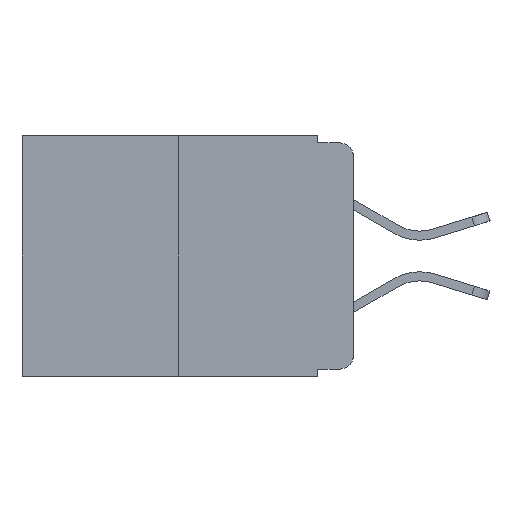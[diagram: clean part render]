
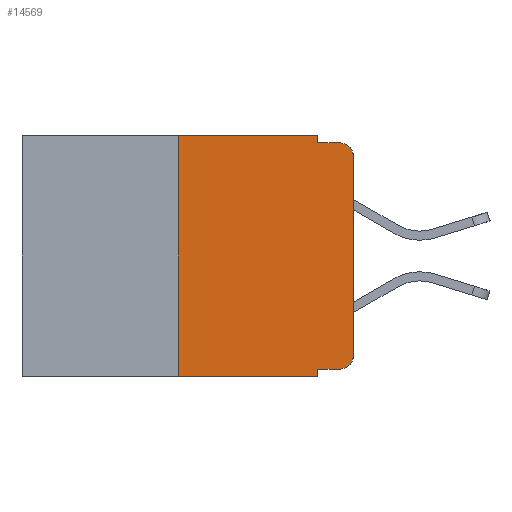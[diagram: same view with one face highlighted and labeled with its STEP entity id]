
A CAD part, left-side view. The second image highlights one B-rep face of the part: STEP entity #14569.
In plain terms, the highlighted planar face has unit normal (-1, 0, 0).
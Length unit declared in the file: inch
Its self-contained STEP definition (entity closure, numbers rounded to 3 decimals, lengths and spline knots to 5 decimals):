
#28 = VECTOR ( 'NONE', #1936, 39.37008 ) ;
#197 = DIRECTION ( 'NONE',  ( 0., 0., -1. ) ) ;
#256 = CARTESIAN_POINT ( 'NONE',  ( 0., 0.02, -0.313 ) ) ;
#475 = VECTOR ( 'NONE', #15218, 39.37008 ) ;
#536 = PLANE ( 'NONE',  #572 ) ;
#572 = AXIS2_PLACEMENT_3D ( 'NONE', #13482, #4297, #12432 ) ;
#718 = EDGE_CURVE ( 'NONE', #2186, #5644, #10550, .T. ) ;
#736 = VERTEX_POINT ( 'NONE', #10210 ) ;
#752 = LINE ( 'NONE', #10221, #3677 ) ;
#781 = LINE ( 'NONE', #7168, #12965 ) ;
#795 = ORIENTED_EDGE ( 'NONE', *, *, #718, .T. ) ;
#831 = ORIENTED_EDGE ( 'NONE', *, *, #15114, .T. ) ;
#867 = ORIENTED_EDGE ( 'NONE', *, *, #14377, .F. ) ;
#888 = ORIENTED_EDGE ( 'NONE', *, *, #13630, .F. ) ;
#1023 = ORIENTED_EDGE ( 'NONE', *, *, #5543, .F. ) ;
#1114 = ORIENTED_EDGE ( 'NONE', *, *, #12880, .F. ) ;
#1164 = ORIENTED_EDGE ( 'NONE', *, *, #5335, .T. ) ;
#1300 = ORIENTED_EDGE ( 'NONE', *, *, #12161, .F. ) ;
#1325 = ORIENTED_EDGE ( 'NONE', *, *, #11409, .T. ) ;
#1339 = ORIENTED_EDGE ( 'NONE', *, *, #10626, .T. ) ;
#1481 = VECTOR ( 'NONE', #7844, 39.37008 ) ;
#1498 = VERTEX_POINT ( 'NONE', #3362 ) ;
#1602 = DIRECTION ( 'NONE',  ( 0., 0., -1. ) ) ;
#1936 = DIRECTION ( 'NONE',  ( 0., -1., 0. ) ) ;
#2186 = VERTEX_POINT ( 'NONE', #4546 ) ;
#2909 = DIRECTION ( 'NONE',  ( -1., 0., 0. ) ) ;
#3362 = CARTESIAN_POINT ( 'NONE',  ( 0., 0.051, 0. ) ) ;
#3677 = VECTOR ( 'NONE', #11398, 39.37008 ) ;
#3698 = CARTESIAN_POINT ( 'NONE',  ( 0., 0.051, -0.343 ) ) ;
#3816 = LINE ( 'NONE', #7253, #475 ) ;
#4297 = DIRECTION ( 'NONE',  ( 1., 0., 0. ) ) ;
#4332 = CARTESIAN_POINT ( 'NONE',  ( 0., 0., 0. ) ) ;
#4421 = CARTESIAN_POINT ( 'NONE',  ( 0., 0.051, -0.333 ) ) ;
#4546 = CARTESIAN_POINT ( 'NONE',  ( 0., 0., -0.313 ) ) ;
#4893 = VECTOR ( 'NONE', #197, 39.37008 ) ;
#4953 = EDGE_LOOP ( 'NONE', ( #795, #831, #867, #888, #1023, #1114, #1164, #1300, #1325, #1339 ) ) ;
#5335 = EDGE_CURVE ( 'NONE', #12653, #10028, #8553, .T. ) ;
#5543 = EDGE_CURVE ( 'NONE', #13305, #1498, #6194, .T. ) ;
#5644 = VERTEX_POINT ( 'NONE', #13742 ) ;
#5685 = DIRECTION ( 'NONE',  ( 0., 0., -1. ) ) ;
#5797 = VERTEX_POINT ( 'NONE', #6253 ) ;
#6194 = LINE ( 'NONE', #10195, #28 ) ;
#6253 = CARTESIAN_POINT ( 'NONE',  ( 0., 0.051, -0.01 ) ) ;
#7168 = CARTESIAN_POINT ( 'NONE',  ( 0., 0.051, -0.01 ) ) ;
#7253 = CARTESIAN_POINT ( 'NONE',  ( 0., 0.25, 0. ) ) ;
#7499 = CARTESIAN_POINT ( 'NONE',  ( 0., 0.473, -0.343 ) ) ;
#7844 = DIRECTION ( 'NONE',  ( 0., 0., 1. ) ) ;
#7954 = CARTESIAN_POINT ( 'NONE',  ( 0., 0.25, -0.343 ) ) ;
#8298 = DIRECTION ( 'NONE',  ( 0., -1., 0. ) ) ;
#8431 = VERTEX_POINT ( 'NONE', #4421 ) ;
#8553 = LINE ( 'NONE', #7499, #14278 ) ;
#8588 = VECTOR ( 'NONE', #5685, 39.37008 ) ;
#8643 = CARTESIAN_POINT ( 'NONE',  ( 0., 0.051, 0. ) ) ;
#8691 = DIRECTION ( 'NONE',  ( -1., 0., 0. ) ) ;
#8816 = VERTEX_POINT ( 'NONE', #13197 ) ;
#9214 = CARTESIAN_POINT ( 'NONE',  ( 0., 0.25, 0. ) ) ;
#9910 = AXIS2_PLACEMENT_3D ( 'NONE', #9954, #2909, #11131 ) ;
#9954 = CARTESIAN_POINT ( 'NONE',  ( 0., 0.02, -0.03 ) ) ;
#9956 = AXIS2_PLACEMENT_3D ( 'NONE', #256, #8691, #1602 ) ;
#10028 = VERTEX_POINT ( 'NONE', #3698 ) ;
#10195 = CARTESIAN_POINT ( 'NONE',  ( 0., 0.473, 0. ) ) ;
#10210 = CARTESIAN_POINT ( 'NONE',  ( 0., 0.02, -0.333 ) ) ;
#10221 = CARTESIAN_POINT ( 'NONE',  ( 0., 0.051, -0.333 ) ) ;
#10550 = LINE ( 'NONE', #4332, #1481 ) ;
#10626 = EDGE_CURVE ( 'NONE', #736, #2186, #14966, .T. ) ;
#10758 = LINE ( 'NONE', #8643, #4893 ) ;
#11131 = DIRECTION ( 'NONE',  ( 0., 0., -1. ) ) ;
#11398 = DIRECTION ( 'NONE',  ( 0., -1., 0. ) ) ;
#11409 = EDGE_CURVE ( 'NONE', #8431, #736, #752, .T. ) ;
#12089 = CIRCLE ( 'NONE', #9910, 0.02 ) ;
#12161 = EDGE_CURVE ( 'NONE', #8431, #10028, #14651, .T. ) ;
#12432 = DIRECTION ( 'NONE',  ( 0., 0., -1. ) ) ;
#12630 = CARTESIAN_POINT ( 'NONE',  ( 0., 0.051, 0. ) ) ;
#12653 = VERTEX_POINT ( 'NONE', #7954 ) ;
#12880 = EDGE_CURVE ( 'NONE', #12653, #13305, #3816, .T. ) ;
#12965 = VECTOR ( 'NONE', #8298, 39.37008 ) ;
#13197 = CARTESIAN_POINT ( 'NONE',  ( 0., 0.02, -0.01 ) ) ;
#13305 = VERTEX_POINT ( 'NONE', #9214 ) ;
#13482 = CARTESIAN_POINT ( 'NONE',  ( 0., 0.473, 0. ) ) ;
#13630 = EDGE_CURVE ( 'NONE', #1498, #5797, #10758, .T. ) ;
#13742 = CARTESIAN_POINT ( 'NONE',  ( 0., 0., -0.03 ) ) ;
#13824 = FACE_OUTER_BOUND ( 'NONE', #4953, .T. ) ;
#14278 = VECTOR ( 'NONE', #14335, 39.37008 ) ;
#14335 = DIRECTION ( 'NONE',  ( 0., -1., 0. ) ) ;
#14377 = EDGE_CURVE ( 'NONE', #5797, #8816, #781, .T. ) ;
#14569 = ADVANCED_FACE ( 'NONE', ( #13824 ), #536, .F. ) ;
#14651 = LINE ( 'NONE', #12630, #8588 ) ;
#14966 = CIRCLE ( 'NONE', #9956, 0.02 ) ;
#15114 = EDGE_CURVE ( 'NONE', #5644, #8816, #12089, .T. ) ;
#15218 = DIRECTION ( 'NONE',  ( 0., 0., 1. ) ) ;
